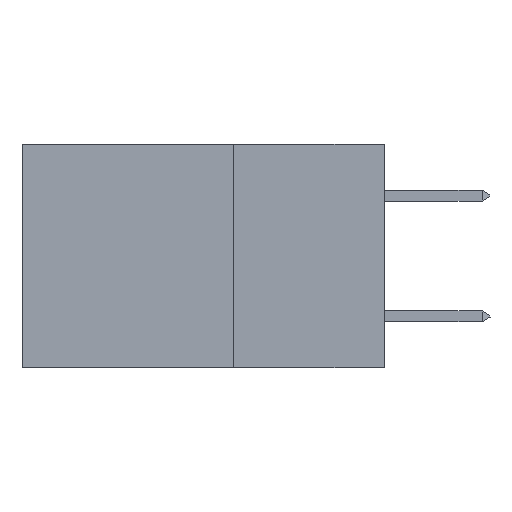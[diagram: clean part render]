
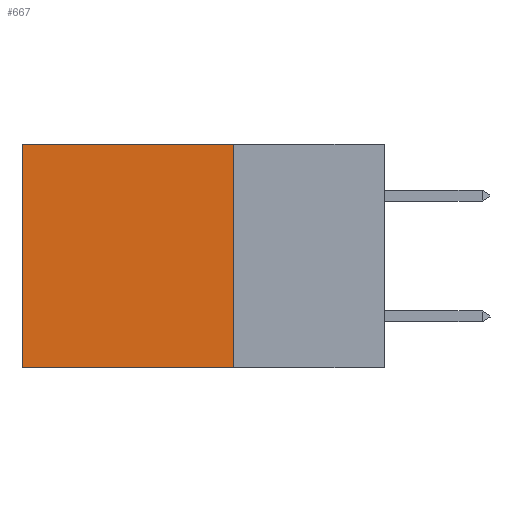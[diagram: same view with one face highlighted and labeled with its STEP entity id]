
A CAD part, left-side view. The second image highlights one B-rep face of the part: STEP entity #667.
In plain terms, the highlighted planar face has unit normal (-1, 0, 0).
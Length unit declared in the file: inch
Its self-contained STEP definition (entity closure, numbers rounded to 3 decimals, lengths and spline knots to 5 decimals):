
#383 = ORIENTED_EDGE ( 'NONE', *, *, #21621, .T. ) ;
#454 = VECTOR ( 'NONE', #21854, 39.37008 ) ;
#653 = DIRECTION ( 'NONE',  ( 0., 0., -1. ) ) ;
#667 = ADVANCED_FACE ( 'NONE', ( #7438 ), #9714, .F. ) ;
#1133 = ORIENTED_EDGE ( 'NONE', *, *, #19629, .F. ) ;
#1449 = CARTESIAN_POINT ( 'NONE',  ( 0.2875, 0.25, -0.37 ) ) ;
#1597 = LINE ( 'NONE', #13226, #21142 ) ;
#1762 = CARTESIAN_POINT ( 'NONE',  ( 0.2875, 0.6, 0. ) ) ;
#6074 = EDGE_CURVE ( 'NONE', #12393, #23557, #10527, .T. ) ;
#7438 = FACE_OUTER_BOUND ( 'NONE', #7449, .T. ) ;
#7449 = EDGE_LOOP ( 'NONE', ( #19471, #1133, #19202, #383 ) ) ;
#7464 = VECTOR ( 'NONE', #13466, 39.37008 ) ;
#8225 = DIRECTION ( 'NONE',  ( 0., 0., -1. ) ) ;
#9653 = LINE ( 'NONE', #12012, #10887 ) ;
#9714 = PLANE ( 'NONE',  #11404 ) ;
#9993 = CARTESIAN_POINT ( 'NONE',  ( 0.2875, 0.25, 0. ) ) ;
#10527 = LINE ( 'NONE', #1762, #454 ) ;
#10887 = VECTOR ( 'NONE', #653, 39.37008 ) ;
#11404 = AXIS2_PLACEMENT_3D ( 'NONE', #16837, #19466, #8225 ) ;
#12012 = CARTESIAN_POINT ( 'NONE',  ( 0.2875, 0.25, 0. ) ) ;
#12393 = VERTEX_POINT ( 'NONE', #14537 ) ;
#13226 = CARTESIAN_POINT ( 'NONE',  ( 0.2875, 0.25, -0.37 ) ) ;
#13466 = DIRECTION ( 'NONE',  ( 0., 1., 0. ) ) ;
#14537 = CARTESIAN_POINT ( 'NONE',  ( 0.2875, 0.6, 0. ) ) ;
#15603 = CARTESIAN_POINT ( 'NONE',  ( 0.2875, 0.25, 0. ) ) ;
#16837 = CARTESIAN_POINT ( 'NONE',  ( 0.2875, 0.25, 0. ) ) ;
#19202 = ORIENTED_EDGE ( 'NONE', *, *, #24312, .F. ) ;
#19466 = DIRECTION ( 'NONE',  ( 1., 0., 0. ) ) ;
#19471 = ORIENTED_EDGE ( 'NONE', *, *, #6074, .T. ) ;
#19629 = EDGE_CURVE ( 'NONE', #23894, #23557, #1597, .T. ) ;
#21142 = VECTOR ( 'NONE', #22691, 39.37008 ) ;
#21325 = CARTESIAN_POINT ( 'NONE',  ( 0.2875, 0.6, -0.37 ) ) ;
#21621 = EDGE_CURVE ( 'NONE', #22348, #12393, #23741, .T. ) ;
#21854 = DIRECTION ( 'NONE',  ( 0., 0., -1. ) ) ;
#22348 = VERTEX_POINT ( 'NONE', #15603 ) ;
#22691 = DIRECTION ( 'NONE',  ( 0., 1., 0. ) ) ;
#23557 = VERTEX_POINT ( 'NONE', #21325 ) ;
#23741 = LINE ( 'NONE', #9993, #7464 ) ;
#23894 = VERTEX_POINT ( 'NONE', #1449 ) ;
#24312 = EDGE_CURVE ( 'NONE', #22348, #23894, #9653, .T. ) ;
